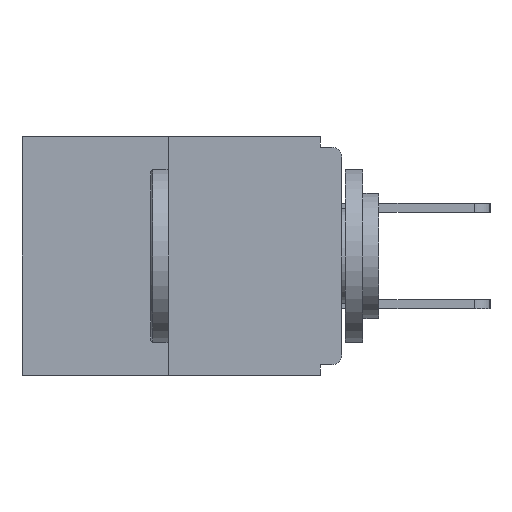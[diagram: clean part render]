
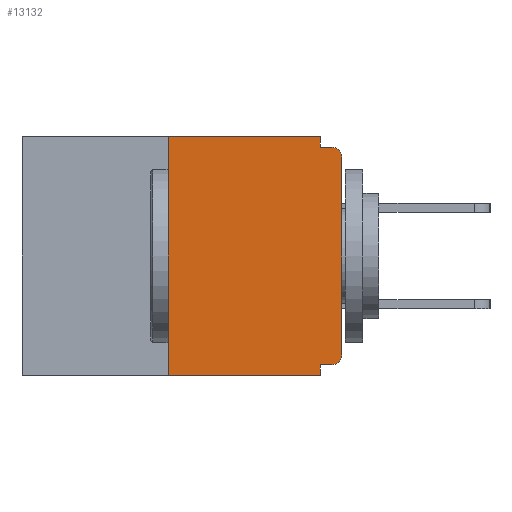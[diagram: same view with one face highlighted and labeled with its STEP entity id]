
A CAD part, left-side view. The second image highlights one B-rep face of the part: STEP entity #13132.
In plain terms, the highlighted planar face has unit normal (-1, 0, 0).
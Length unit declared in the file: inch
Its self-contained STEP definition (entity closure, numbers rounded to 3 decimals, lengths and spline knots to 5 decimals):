
#251 = AXIS2_PLACEMENT_3D ( 'NONE', #3818, #13996, #7249 ) ;
#357 = VECTOR ( 'NONE', #8967, 39.37008 ) ;
#552 = LINE ( 'NONE', #8000, #4149 ) ;
#653 = EDGE_CURVE ( 'NONE', #13327, #1512, #9558, .T. ) ;
#686 = CARTESIAN_POINT ( 'NONE',  ( 0., 0.46, 0. ) ) ;
#702 = ORIENTED_EDGE ( 'NONE', *, *, #12437, .T. ) ;
#706 = LINE ( 'NONE', #14607, #357 ) ;
#778 = DIRECTION ( 'NONE',  ( 1., 0., 0. ) ) ;
#1076 = DIRECTION ( 'NONE',  ( 0., 0., -1. ) ) ;
#1093 = CARTESIAN_POINT ( 'NONE',  ( 0., 0.031, 0. ) ) ;
#1181 = VECTOR ( 'NONE', #2681, 39.37008 ) ;
#1197 = DIRECTION ( 'NONE',  ( 0., -1., 0. ) ) ;
#1448 = VERTEX_POINT ( 'NONE', #3047 ) ;
#1512 = VERTEX_POINT ( 'NONE', #11384 ) ;
#1616 = CARTESIAN_POINT ( 'NONE',  ( 0., 0.46, -0.343 ) ) ;
#2041 = EDGE_CURVE ( 'NONE', #8391, #13327, #5398, .T. ) ;
#2185 = EDGE_CURVE ( 'NONE', #9680, #1448, #706, .T. ) ;
#2623 = ORIENTED_EDGE ( 'NONE', *, *, #13251, .F. ) ;
#2681 = DIRECTION ( 'NONE',  ( 0., -1., 0. ) ) ;
#2730 = ORIENTED_EDGE ( 'NONE', *, *, #3954, .F. ) ;
#2768 = ORIENTED_EDGE ( 'NONE', *, *, #8698, .T. ) ;
#3041 = DIRECTION ( 'NONE',  ( 0., 0., -1. ) ) ;
#3047 = CARTESIAN_POINT ( 'NONE',  ( 0., 0., -0.03 ) ) ;
#3154 = LINE ( 'NONE', #3434, #13811 ) ;
#3270 = DIRECTION ( 'NONE',  ( 0., 0., 1. ) ) ;
#3434 = CARTESIAN_POINT ( 'NONE',  ( 0., 0., -0.328 ) ) ;
#3461 = CARTESIAN_POINT ( 'NONE',  ( 0., 0.015, -0.015 ) ) ;
#3667 = FACE_OUTER_BOUND ( 'NONE', #13725, .T. ) ;
#3818 = CARTESIAN_POINT ( 'NONE',  ( 0., 0.015, -0.313 ) ) ;
#3954 = EDGE_CURVE ( 'NONE', #7344, #14171, #3154, .T. ) ;
#4149 = VECTOR ( 'NONE', #3270, 39.37008 ) ;
#4196 = DIRECTION ( 'NONE',  ( 0., 0., -1. ) ) ;
#4247 = PLANE ( 'NONE',  #6537 ) ;
#4466 = ORIENTED_EDGE ( 'NONE', *, *, #2041, .F. ) ;
#4495 = CARTESIAN_POINT ( 'NONE',  ( 0., 0.25, 0. ) ) ;
#4794 = LINE ( 'NONE', #1616, #1181 ) ;
#5034 = VECTOR ( 'NONE', #6234, 39.37008 ) ;
#5216 = VECTOR ( 'NONE', #1197, 39.37008 ) ;
#5398 = LINE ( 'NONE', #6929, #5216 ) ;
#5435 = VERTEX_POINT ( 'NONE', #12996 ) ;
#5547 = ORIENTED_EDGE ( 'NONE', *, *, #9775, .T. ) ;
#6234 = DIRECTION ( 'NONE',  ( 0., -1., 0. ) ) ;
#6537 = AXIS2_PLACEMENT_3D ( 'NONE', #686, #778, #4196 ) ;
#6681 = ORIENTED_EDGE ( 'NONE', *, *, #2185, .T. ) ;
#6710 = CARTESIAN_POINT ( 'NONE',  ( 0., 0., -0.313 ) ) ;
#6822 = EDGE_CURVE ( 'NONE', #9965, #8391, #552, .T. ) ;
#6929 = CARTESIAN_POINT ( 'NONE',  ( 0., 0.46, 0. ) ) ;
#7163 = ORIENTED_EDGE ( 'NONE', *, *, #653, .F. ) ;
#7249 = DIRECTION ( 'NONE',  ( 0., 0., -1. ) ) ;
#7286 = CARTESIAN_POINT ( 'NONE',  ( 0., 0.25, -0.343 ) ) ;
#7311 = CARTESIAN_POINT ( 'NONE',  ( 0., 0.031, 0. ) ) ;
#7344 = VERTEX_POINT ( 'NONE', #7537 ) ;
#7395 = ORIENTED_EDGE ( 'NONE', *, *, #11183, .F. ) ;
#7537 = CARTESIAN_POINT ( 'NONE',  ( 0., 0.015, -0.328 ) ) ;
#7857 = CARTESIAN_POINT ( 'NONE',  ( 0., 0.031, -0.343 ) ) ;
#7864 = LINE ( 'NONE', #9738, #5034 ) ;
#8000 = CARTESIAN_POINT ( 'NONE',  ( 0., 0.25, 0. ) ) ;
#8391 = VERTEX_POINT ( 'NONE', #4495 ) ;
#8620 = CIRCLE ( 'NONE', #251, 0.015 ) ;
#8632 = DIRECTION ( 'NONE',  ( 0., 0., -1. ) ) ;
#8698 = EDGE_CURVE ( 'NONE', #1448, #11912, #11833, .T. ) ;
#8874 = VECTOR ( 'NONE', #1076, 39.37008 ) ;
#8967 = DIRECTION ( 'NONE',  ( 0., 0., 1. ) ) ;
#9352 = AXIS2_PLACEMENT_3D ( 'NONE', #13157, #14238, #8632 ) ;
#9558 = LINE ( 'NONE', #1093, #11669 ) ;
#9680 = VERTEX_POINT ( 'NONE', #6710 ) ;
#9738 = CARTESIAN_POINT ( 'NONE',  ( 0., 0., -0.015 ) ) ;
#9740 = LINE ( 'NONE', #7857, #8874 ) ;
#9775 = EDGE_CURVE ( 'NONE', #7344, #9680, #8620, .T. ) ;
#9965 = VERTEX_POINT ( 'NONE', #7286 ) ;
#10445 = ORIENTED_EDGE ( 'NONE', *, *, #6822, .F. ) ;
#10556 = CARTESIAN_POINT ( 'NONE',  ( 0., 0.031, -0.328 ) ) ;
#11183 = EDGE_CURVE ( 'NONE', #1512, #11912, #7864, .T. ) ;
#11384 = CARTESIAN_POINT ( 'NONE',  ( 0., 0.031, -0.015 ) ) ;
#11669 = VECTOR ( 'NONE', #3041, 39.37008 ) ;
#11833 = CIRCLE ( 'NONE', #9352, 0.015 ) ;
#11912 = VERTEX_POINT ( 'NONE', #3461 ) ;
#12437 = EDGE_CURVE ( 'NONE', #9965, #5435, #4794, .T. ) ;
#12996 = CARTESIAN_POINT ( 'NONE',  ( 0., 0.031, -0.343 ) ) ;
#13132 = ADVANCED_FACE ( 'NONE', ( #3667 ), #4247, .F. ) ;
#13157 = CARTESIAN_POINT ( 'NONE',  ( 0., 0.015, -0.03 ) ) ;
#13251 = EDGE_CURVE ( 'NONE', #14171, #5435, #9740, .T. ) ;
#13327 = VERTEX_POINT ( 'NONE', #7311 ) ;
#13568 = DIRECTION ( 'NONE',  ( 0., 1., 0. ) ) ;
#13725 = EDGE_LOOP ( 'NONE', ( #4466, #10445, #702, #2623, #2730, #5547, #6681, #2768, #7395, #7163 ) ) ;
#13811 = VECTOR ( 'NONE', #13568, 39.37008 ) ;
#13996 = DIRECTION ( 'NONE',  ( -1., 0., 0. ) ) ;
#14171 = VERTEX_POINT ( 'NONE', #10556 ) ;
#14238 = DIRECTION ( 'NONE',  ( -1., 0., 0. ) ) ;
#14607 = CARTESIAN_POINT ( 'NONE',  ( 0., 0., 0. ) ) ;
